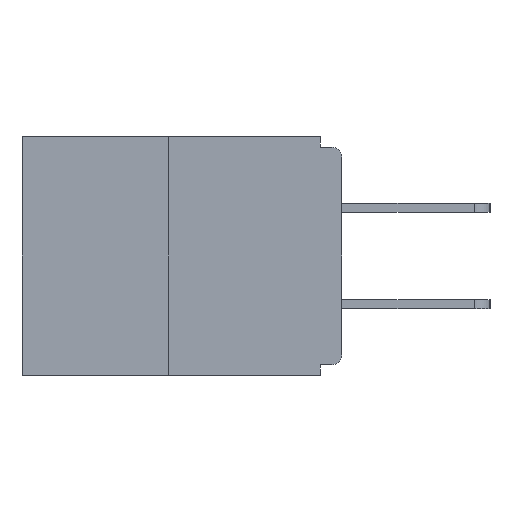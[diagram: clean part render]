
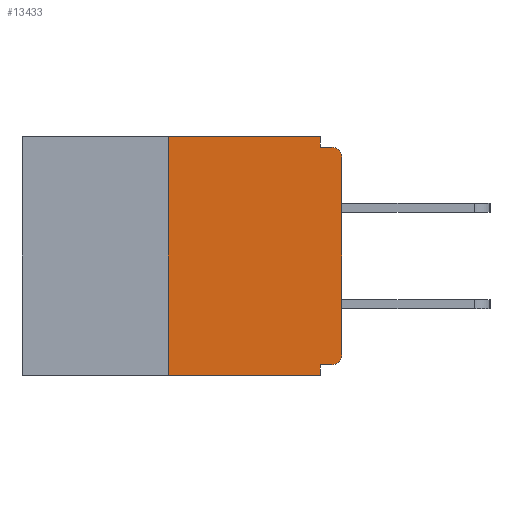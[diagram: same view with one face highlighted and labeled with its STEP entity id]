
A CAD part, left-side view. The second image highlights one B-rep face of the part: STEP entity #13433.
In plain terms, the highlighted planar face has unit normal (-1, 0, 0).
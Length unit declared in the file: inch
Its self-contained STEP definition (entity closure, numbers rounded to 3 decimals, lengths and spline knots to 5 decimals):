
#21 = EDGE_LOOP ( 'NONE', ( #19190, #7913, #15805, #14105, #2224, #20160, #25246, #4229, #23966, #9325 ) ) ;
#351 = EDGE_CURVE ( 'NONE', #25797, #3941, #19214, .T. ) ;
#509 = EDGE_CURVE ( 'NONE', #17894, #25797, #7288, .T. ) ;
#565 = VECTOR ( 'NONE', #13918, 39.37008 ) ;
#1303 = VECTOR ( 'NONE', #19924, 39.37008 ) ;
#1462 = CARTESIAN_POINT ( 'NONE',  ( 0., 0.015, -0.328 ) ) ;
#2224 = ORIENTED_EDGE ( 'NONE', *, *, #14296, .F. ) ;
#3230 = DIRECTION ( 'NONE',  ( 0., 0., -1. ) ) ;
#3279 = EDGE_CURVE ( 'NONE', #5568, #10861, #8734, .T. ) ;
#3941 = VERTEX_POINT ( 'NONE', #16936 ) ;
#3950 = DIRECTION ( 'NONE',  ( -1., 0., 0. ) ) ;
#4021 = LINE ( 'NONE', #11241, #11019 ) ;
#4229 = ORIENTED_EDGE ( 'NONE', *, *, #351, .T. ) ;
#4384 = CARTESIAN_POINT ( 'NONE',  ( 0., 0.46, 0. ) ) ;
#4683 = CIRCLE ( 'NONE', #22941, 0.015 ) ;
#5568 = VERTEX_POINT ( 'NONE', #17976 ) ;
#5884 = VECTOR ( 'NONE', #15995, 39.37008 ) ;
#5886 = LINE ( 'NONE', #12817, #1303 ) ;
#6102 = CARTESIAN_POINT ( 'NONE',  ( 0., 0.015, -0.03 ) ) ;
#6220 = CARTESIAN_POINT ( 'NONE',  ( 0., 0.015, -0.313 ) ) ;
#7288 = LINE ( 'NONE', #26073, #565 ) ;
#7306 = VERTEX_POINT ( 'NONE', #27347 ) ;
#7819 = CARTESIAN_POINT ( 'NONE',  ( 0., 0.031, 0. ) ) ;
#7840 = VERTEX_POINT ( 'NONE', #13702 ) ;
#7913 = ORIENTED_EDGE ( 'NONE', *, *, #9818, .F. ) ;
#8734 = LINE ( 'NONE', #18590, #5884 ) ;
#9325 = ORIENTED_EDGE ( 'NONE', *, *, #25133, .F. ) ;
#9818 = EDGE_CURVE ( 'NONE', #15850, #7306, #5886, .T. ) ;
#10082 = CARTESIAN_POINT ( 'NONE',  ( 0., 0.031, -0.015 ) ) ;
#10410 = AXIS2_PLACEMENT_3D ( 'NONE', #6102, #3950, #13487 ) ;
#10861 = VERTEX_POINT ( 'NONE', #19028 ) ;
#11019 = VECTOR ( 'NONE', #16034, 39.37008 ) ;
#11241 = CARTESIAN_POINT ( 'NONE',  ( 0., 0., -0.015 ) ) ;
#11309 = FACE_OUTER_BOUND ( 'NONE', #21, .T. ) ;
#11869 = EDGE_CURVE ( 'NONE', #15850, #10861, #16882, .T. ) ;
#12467 = EDGE_CURVE ( 'NONE', #28078, #3941, #4021, .T. ) ;
#12817 = CARTESIAN_POINT ( 'NONE',  ( 0., 0.25, 0. ) ) ;
#13298 = DIRECTION ( 'NONE',  ( -1., 0., 0. ) ) ;
#13433 = ADVANCED_FACE ( 'NONE', ( #11309 ), #28094, .F. ) ;
#13487 = DIRECTION ( 'NONE',  ( 0., 0., -1. ) ) ;
#13702 = CARTESIAN_POINT ( 'NONE',  ( 0., 0.031, 0. ) ) ;
#13918 = DIRECTION ( 'NONE',  ( 0., 0., 1. ) ) ;
#13920 = LINE ( 'NONE', #23342, #25413 ) ;
#14105 = ORIENTED_EDGE ( 'NONE', *, *, #3279, .F. ) ;
#14296 = EDGE_CURVE ( 'NONE', #14770, #5568, #15187, .T. ) ;
#14391 = VECTOR ( 'NONE', #21657, 39.37008 ) ;
#14770 = VERTEX_POINT ( 'NONE', #1462 ) ;
#15187 = LINE ( 'NONE', #22298, #19456 ) ;
#15649 = CARTESIAN_POINT ( 'NONE',  ( 0., 0., -0.313 ) ) ;
#15805 = ORIENTED_EDGE ( 'NONE', *, *, #11869, .T. ) ;
#15850 = VERTEX_POINT ( 'NONE', #26812 ) ;
#15995 = DIRECTION ( 'NONE',  ( 0., 0., -1. ) ) ;
#16034 = DIRECTION ( 'NONE',  ( 0., -1., 0. ) ) ;
#16104 = DIRECTION ( 'NONE',  ( 0., 0., -1. ) ) ;
#16479 = AXIS2_PLACEMENT_3D ( 'NONE', #4384, #27948, #16104 ) ;
#16882 = LINE ( 'NONE', #26270, #14391 ) ;
#16936 = CARTESIAN_POINT ( 'NONE',  ( 0., 0.015, -0.015 ) ) ;
#17894 = VERTEX_POINT ( 'NONE', #15649 ) ;
#17976 = CARTESIAN_POINT ( 'NONE',  ( 0., 0.031, -0.328 ) ) ;
#18065 = EDGE_CURVE ( 'NONE', #7306, #7840, #13920, .T. ) ;
#18590 = CARTESIAN_POINT ( 'NONE',  ( 0., 0.031, -0.343 ) ) ;
#19028 = CARTESIAN_POINT ( 'NONE',  ( 0., 0.031, -0.343 ) ) ;
#19190 = ORIENTED_EDGE ( 'NONE', *, *, #18065, .F. ) ;
#19214 = CIRCLE ( 'NONE', #10410, 0.015 ) ;
#19456 = VECTOR ( 'NONE', #24596, 39.37008 ) ;
#19924 = DIRECTION ( 'NONE',  ( 0., 0., 1. ) ) ;
#20019 = LINE ( 'NONE', #7819, #21746 ) ;
#20160 = ORIENTED_EDGE ( 'NONE', *, *, #28712, .T. ) ;
#20396 = DIRECTION ( 'NONE',  ( 0., 0., -1. ) ) ;
#20681 = CARTESIAN_POINT ( 'NONE',  ( 0., 0., -0.03 ) ) ;
#21031 = DIRECTION ( 'NONE',  ( 0., -1., 0. ) ) ;
#21657 = DIRECTION ( 'NONE',  ( 0., -1., 0. ) ) ;
#21746 = VECTOR ( 'NONE', #3230, 39.37008 ) ;
#22298 = CARTESIAN_POINT ( 'NONE',  ( 0., 0., -0.328 ) ) ;
#22941 = AXIS2_PLACEMENT_3D ( 'NONE', #6220, #13298, #20396 ) ;
#23342 = CARTESIAN_POINT ( 'NONE',  ( 0., 0.46, 0. ) ) ;
#23966 = ORIENTED_EDGE ( 'NONE', *, *, #12467, .F. ) ;
#24596 = DIRECTION ( 'NONE',  ( 0., 1., 0. ) ) ;
#25133 = EDGE_CURVE ( 'NONE', #7840, #28078, #20019, .T. ) ;
#25246 = ORIENTED_EDGE ( 'NONE', *, *, #509, .T. ) ;
#25413 = VECTOR ( 'NONE', #21031, 39.37008 ) ;
#25797 = VERTEX_POINT ( 'NONE', #20681 ) ;
#26073 = CARTESIAN_POINT ( 'NONE',  ( 0., 0., 0. ) ) ;
#26270 = CARTESIAN_POINT ( 'NONE',  ( 0., 0.46, -0.343 ) ) ;
#26812 = CARTESIAN_POINT ( 'NONE',  ( 0., 0.25, -0.343 ) ) ;
#27347 = CARTESIAN_POINT ( 'NONE',  ( 0., 0.25, 0. ) ) ;
#27948 = DIRECTION ( 'NONE',  ( 1., 0., 0. ) ) ;
#28078 = VERTEX_POINT ( 'NONE', #10082 ) ;
#28094 = PLANE ( 'NONE',  #16479 ) ;
#28712 = EDGE_CURVE ( 'NONE', #14770, #17894, #4683, .T. ) ;
